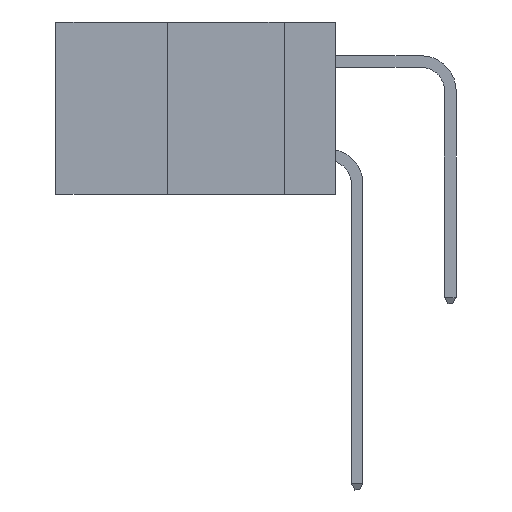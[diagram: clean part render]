
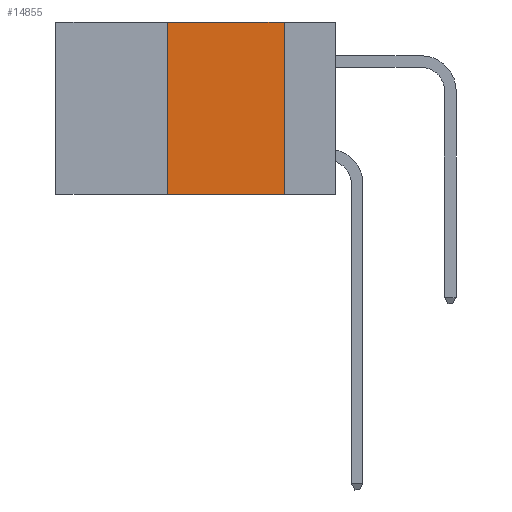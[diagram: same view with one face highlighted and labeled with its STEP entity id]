
A CAD part, left-side view. The second image highlights one B-rep face of the part: STEP entity #14855.
In plain terms, the highlighted planar face has unit normal (-1, 0, 0).
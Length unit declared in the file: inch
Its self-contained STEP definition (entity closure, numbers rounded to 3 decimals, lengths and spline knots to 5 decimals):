
#499 = CARTESIAN_POINT ( 'NONE',  ( 0., 0.36, 0. ) ) ;
#507 = CARTESIAN_POINT ( 'NONE',  ( 0., 0.6, -0.37 ) ) ;
#596 = VERTEX_POINT ( 'NONE', #6005 ) ;
#2220 = DIRECTION ( 'NONE',  ( 1., 0., 0. ) ) ;
#3002 = CARTESIAN_POINT ( 'NONE',  ( 0., 0.6, 0. ) ) ;
#3093 = LINE ( 'NONE', #3002, #4819 ) ;
#3968 = CARTESIAN_POINT ( 'NONE',  ( 0., 0.36, 0. ) ) ;
#4117 = ORIENTED_EDGE ( 'NONE', *, *, #5594, .F. ) ;
#4195 = CARTESIAN_POINT ( 'NONE',  ( 0., 0.36, -0.37 ) ) ;
#4819 = VECTOR ( 'NONE', #16065, 39.37008 ) ;
#5071 = CARTESIAN_POINT ( 'NONE',  ( 0., 0.11, -0.37 ) ) ;
#5575 = LINE ( 'NONE', #499, #6010 ) ;
#5594 = EDGE_CURVE ( 'NONE', #596, #15955, #7427, .T. ) ;
#6005 = CARTESIAN_POINT ( 'NONE',  ( 0., 0.11, 0. ) ) ;
#6010 = VECTOR ( 'NONE', #9364, 39.37008 ) ;
#6334 = EDGE_CURVE ( 'NONE', #16525, #15955, #14934, .T. ) ;
#6846 = ORIENTED_EDGE ( 'NONE', *, *, #6334, .T. ) ;
#7427 = LINE ( 'NONE', #8553, #9260 ) ;
#7630 = EDGE_CURVE ( 'NONE', #14275, #596, #3093, .T. ) ;
#8377 = ORIENTED_EDGE ( 'NONE', *, *, #16551, .F. ) ;
#8553 = CARTESIAN_POINT ( 'NONE',  ( 0., 0.11, 0. ) ) ;
#9260 = VECTOR ( 'NONE', #12662, 39.37008 ) ;
#9364 = DIRECTION ( 'NONE',  ( 0., 0., 1. ) ) ;
#9827 = AXIS2_PLACEMENT_3D ( 'NONE', #16246, #2220, #12546 ) ;
#11025 = PLANE ( 'NONE',  #9827 ) ;
#11782 = ORIENTED_EDGE ( 'NONE', *, *, #7630, .F. ) ;
#12302 = FACE_OUTER_BOUND ( 'NONE', #14699, .T. ) ;
#12546 = DIRECTION ( 'NONE',  ( 0., 0., -1. ) ) ;
#12662 = DIRECTION ( 'NONE',  ( 0., 0., -1. ) ) ;
#13568 = DIRECTION ( 'NONE',  ( 0., -1., 0. ) ) ;
#14275 = VERTEX_POINT ( 'NONE', #3968 ) ;
#14699 = EDGE_LOOP ( 'NONE', ( #4117, #11782, #8377, #6846 ) ) ;
#14855 = ADVANCED_FACE ( 'NONE', ( #12302 ), #11025, .F. ) ;
#14934 = LINE ( 'NONE', #507, #15036 ) ;
#15036 = VECTOR ( 'NONE', #13568, 39.37008 ) ;
#15955 = VERTEX_POINT ( 'NONE', #5071 ) ;
#16065 = DIRECTION ( 'NONE',  ( 0., -1., 0. ) ) ;
#16246 = CARTESIAN_POINT ( 'NONE',  ( 0., 0.6, 0. ) ) ;
#16525 = VERTEX_POINT ( 'NONE', #4195 ) ;
#16551 = EDGE_CURVE ( 'NONE', #16525, #14275, #5575, .T. ) ;
